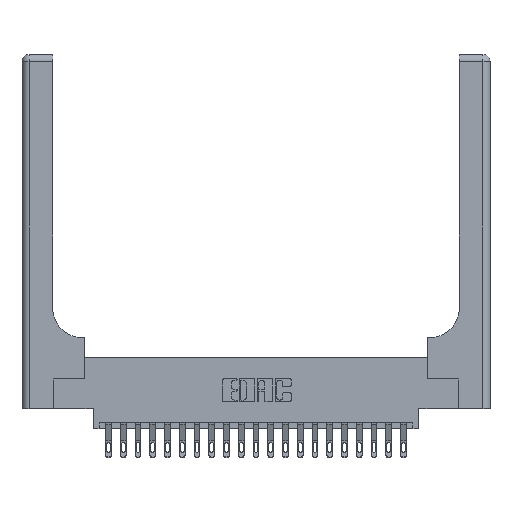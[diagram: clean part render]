
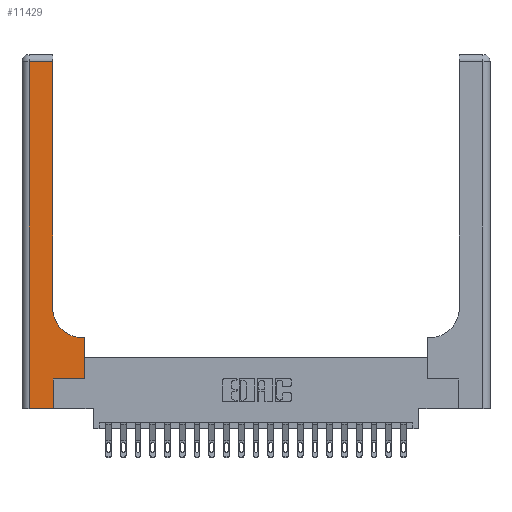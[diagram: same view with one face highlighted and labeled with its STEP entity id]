
A CAD part, top view. The second image highlights one B-rep face of the part: STEP entity #11429.
In plain terms, the highlighted planar face has unit normal (0, 0, 1).
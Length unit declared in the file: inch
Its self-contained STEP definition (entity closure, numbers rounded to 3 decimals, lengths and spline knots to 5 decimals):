
#204 = CIRCLE ( 'NONE', #6079, 0.25 ) ;
#558 = EDGE_CURVE ( 'NONE', #2060, #3040, #14097, .T. ) ;
#613 = CARTESIAN_POINT ( 'NONE',  ( 0., 2.94, 0.37 ) ) ;
#705 = VECTOR ( 'NONE', #8423, 39.37008 ) ;
#1011 = CARTESIAN_POINT ( 'NONE',  ( 0.26, 2.94, 0.37 ) ) ;
#1211 = VERTEX_POINT ( 'NONE', #16569 ) ;
#2060 = VERTEX_POINT ( 'NONE', #9651 ) ;
#2129 = ORIENTED_EDGE ( 'NONE', *, *, #5272, .T. ) ;
#2212 = CARTESIAN_POINT ( 'NONE',  ( 0.51, 0.85, 0.37 ) ) ;
#2681 = VERTEX_POINT ( 'NONE', #6255 ) ;
#3040 = VERTEX_POINT ( 'NONE', #7488 ) ;
#3122 = EDGE_CURVE ( 'NONE', #10723, #8789, #4502, .T. ) ;
#3392 = CARTESIAN_POINT ( 'NONE',  ( 0., 0., 0.37 ) ) ;
#3832 = EDGE_CURVE ( 'NONE', #5473, #2060, #4765, .T. ) ;
#3888 = ORIENTED_EDGE ( 'NONE', *, *, #3832, .T. ) ;
#4029 = VERTEX_POINT ( 'NONE', #21002 ) ;
#4205 = VECTOR ( 'NONE', #7547, 39.37008 ) ;
#4502 = LINE ( 'NONE', #13196, #9859 ) ;
#4765 = LINE ( 'NONE', #3392, #705 ) ;
#5167 = AXIS2_PLACEMENT_3D ( 'NONE', #11895, #15652, #13931 ) ;
#5272 = EDGE_CURVE ( 'NONE', #1211, #5473, #10604, .T. ) ;
#5473 = VERTEX_POINT ( 'NONE', #13655 ) ;
#5547 = ORIENTED_EDGE ( 'NONE', *, *, #3122, .T. ) ;
#5553 = EDGE_CURVE ( 'NONE', #18975, #2681, #17218, .T. ) ;
#5579 = VECTOR ( 'NONE', #21709, 39.37008 ) ;
#5838 = CARTESIAN_POINT ( 'NONE',  ( 0.26, 0.6, 0.37 ) ) ;
#6079 = AXIS2_PLACEMENT_3D ( 'NONE', #2212, #7486, #7030 ) ;
#6109 = CARTESIAN_POINT ( 'NONE',  ( 0.26, 0.85, 0.37 ) ) ;
#6255 = CARTESIAN_POINT ( 'NONE',  ( 0.528, 0.6, 0.37 ) ) ;
#7030 = DIRECTION ( 'NONE',  ( 1., 0., 0. ) ) ;
#7486 = DIRECTION ( 'NONE',  ( 0., 0., -1. ) ) ;
#7488 = CARTESIAN_POINT ( 'NONE',  ( 0.265, 0.25, 0.37 ) ) ;
#7547 = DIRECTION ( 'NONE',  ( -1., 0., 0. ) ) ;
#8423 = DIRECTION ( 'NONE',  ( 1., 0., 0. ) ) ;
#8685 = FACE_OUTER_BOUND ( 'NONE', #12941, .T. ) ;
#8789 = VERTEX_POINT ( 'NONE', #1011 ) ;
#9114 = DIRECTION ( 'NONE',  ( 0., -1., 0. ) ) ;
#9204 = LINE ( 'NONE', #613, #11036 ) ;
#9651 = CARTESIAN_POINT ( 'NONE',  ( 0.265, 0., 0.37 ) ) ;
#9859 = VECTOR ( 'NONE', #11374, 39.37008 ) ;
#10604 = LINE ( 'NONE', #17696, #20071 ) ;
#10723 = VERTEX_POINT ( 'NONE', #6109 ) ;
#11036 = VECTOR ( 'NONE', #16187, 39.37008 ) ;
#11374 = DIRECTION ( 'NONE',  ( 0., 1., 0. ) ) ;
#11429 = ADVANCED_FACE ( 'NONE', ( #8685 ), #20574, .F. ) ;
#11895 = CARTESIAN_POINT ( 'NONE',  ( 0., 3., 0.37 ) ) ;
#11959 = CARTESIAN_POINT ( 'NONE',  ( 0.528, 0.25, 0.37 ) ) ;
#12054 = EDGE_CURVE ( 'NONE', #8789, #1211, #9204, .T. ) ;
#12681 = LINE ( 'NONE', #19646, #5579 ) ;
#12914 = EDGE_CURVE ( 'NONE', #3040, #18975, #12681, .T. ) ;
#12941 = EDGE_LOOP ( 'NONE', ( #5547, #22176, #2129, #3888, #21805, #18466, #17433, #18515, #19365 ) ) ;
#13196 = CARTESIAN_POINT ( 'NONE',  ( 0.26, 3., 0.37 ) ) ;
#13655 = CARTESIAN_POINT ( 'NONE',  ( 0.06, 0., 0.37 ) ) ;
#13931 = DIRECTION ( 'NONE',  ( -1., 0., 0. ) ) ;
#14097 = LINE ( 'NONE', #21087, #22016 ) ;
#15652 = DIRECTION ( 'NONE',  ( 0., 0., -1. ) ) ;
#15765 = CARTESIAN_POINT ( 'NONE',  ( 0.528, 0.25, 0.37 ) ) ;
#16187 = DIRECTION ( 'NONE',  ( -1., 0., 0. ) ) ;
#16569 = CARTESIAN_POINT ( 'NONE',  ( 0.06, 2.94, 0.37 ) ) ;
#16873 = DIRECTION ( 'NONE',  ( 0., 1., 0. ) ) ;
#17218 = LINE ( 'NONE', #11959, #19355 ) ;
#17433 = ORIENTED_EDGE ( 'NONE', *, *, #5553, .T. ) ;
#17667 = DIRECTION ( 'NONE',  ( 0., 1., 0. ) ) ;
#17696 = CARTESIAN_POINT ( 'NONE',  ( 0.06, 3., 0.37 ) ) ;
#18466 = ORIENTED_EDGE ( 'NONE', *, *, #12914, .T. ) ;
#18515 = ORIENTED_EDGE ( 'NONE', *, *, #21096, .T. ) ;
#18975 = VERTEX_POINT ( 'NONE', #15765 ) ;
#19355 = VECTOR ( 'NONE', #16873, 39.37008 ) ;
#19365 = ORIENTED_EDGE ( 'NONE', *, *, #21983, .T. ) ;
#19646 = CARTESIAN_POINT ( 'NONE',  ( 0.265, 0.25, 0.37 ) ) ;
#20071 = VECTOR ( 'NONE', #9114, 39.37008 ) ;
#20574 = PLANE ( 'NONE',  #5167 ) ;
#21002 = CARTESIAN_POINT ( 'NONE',  ( 0.51, 0.6, 0.37 ) ) ;
#21087 = CARTESIAN_POINT ( 'NONE',  ( 0.265, 0., 0.37 ) ) ;
#21096 = EDGE_CURVE ( 'NONE', #2681, #4029, #21375, .T. ) ;
#21375 = LINE ( 'NONE', #5838, #4205 ) ;
#21709 = DIRECTION ( 'NONE',  ( 1., 0., 0. ) ) ;
#21805 = ORIENTED_EDGE ( 'NONE', *, *, #558, .T. ) ;
#21983 = EDGE_CURVE ( 'NONE', #4029, #10723, #204, .T. ) ;
#22016 = VECTOR ( 'NONE', #17667, 39.37008 ) ;
#22176 = ORIENTED_EDGE ( 'NONE', *, *, #12054, .T. ) ;
